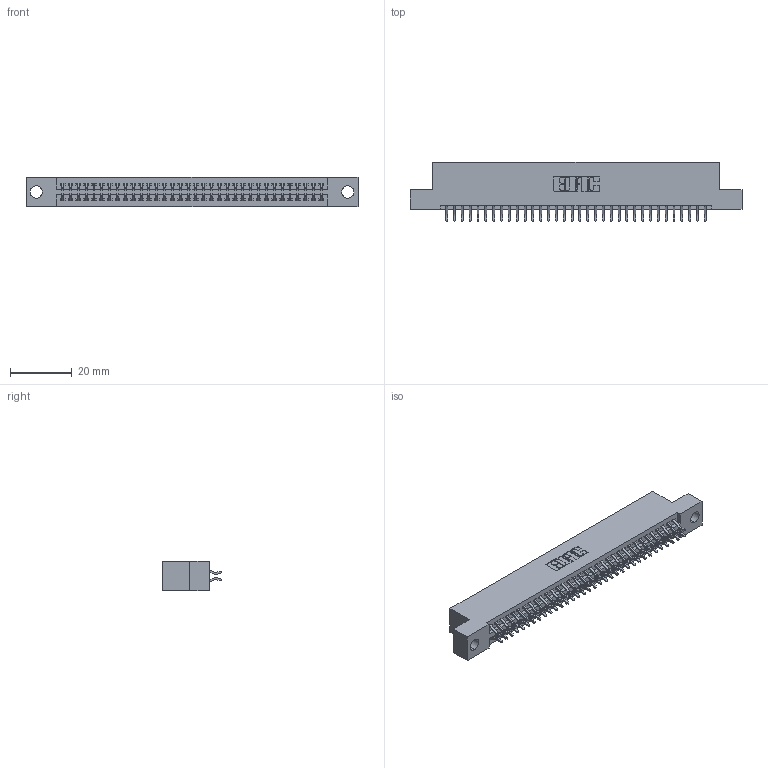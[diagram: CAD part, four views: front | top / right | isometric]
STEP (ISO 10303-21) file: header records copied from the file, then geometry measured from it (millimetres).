
FILE_DESCRIPTION (( 'STEP AP203' ), '1' );
FILE_NAME ('395-068-556-204.STEP', '2021-06-17T04:07:13', ( '' ), ( '' ), 'SwSTEP 2.0', 'SolidWorks 2020', '' );
FILE_SCHEMA (( 'CONFIG_CONTROL_DESIGN' ));
Length unit declared in the file: inch
Products named in the file (3): 395-068-556-204; 345-292-001_556 Tail; 345 Part_Flush Mounting Lugs - 0.156 Dia-TI
Assembly tree (69 placements, depth 2):
  395-068-556-204
    345 Part_Flush Mounting Lugs - 0.156 Dia-TI
    345-292-001_556 Tail  x68
Bounding box: 107.57 x 19.24 x 9.4 mm (x, y, z)
Volume: 10266.5 mm3; surface area: 14812.7 mm2
Topology: 69 solids, 69 shells, 3948 faces, 11733 edges, 7730 vertices
Faces by surface type: plane 2610, cylinder 1338
Entity records: 28393 total; most frequent: CARTESIAN_POINT 4786, ORIENTED_EDGE 4706, DIRECTION 4217, EDGE_CURVE 2353, VECTOR 2077, LINE 2077, VERTEX_POINT 1566, AXIS2_PLACEMENT_3D 1070
